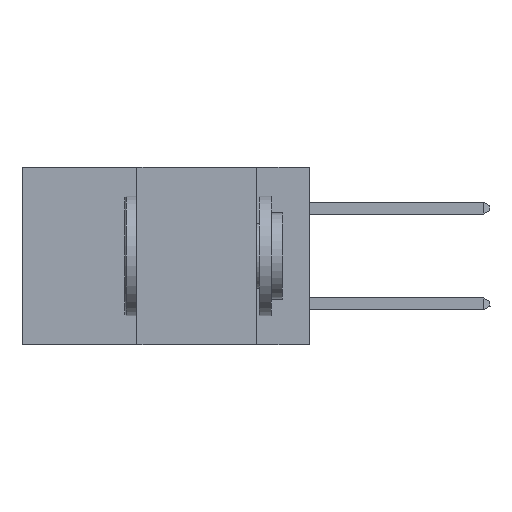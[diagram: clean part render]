
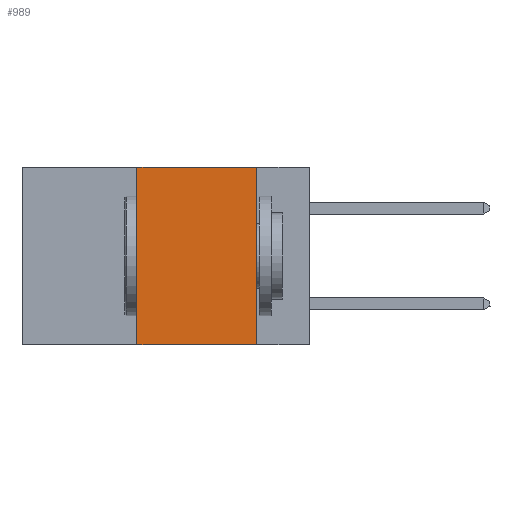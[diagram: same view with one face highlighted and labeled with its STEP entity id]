
A CAD part, left-side view. The second image highlights one B-rep face of the part: STEP entity #989.
In plain terms, the highlighted planar face has unit normal (-1, 0, 0).
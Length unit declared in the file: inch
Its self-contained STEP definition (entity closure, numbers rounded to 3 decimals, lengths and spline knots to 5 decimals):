
#76 = CARTESIAN_POINT ( 'NONE',  ( 0., 0.6, -0.37 ) ) ;
#334 = CARTESIAN_POINT ( 'NONE',  ( 0., 0.6, 0. ) ) ;
#580 = FACE_OUTER_BOUND ( 'NONE', #6560, .T. ) ;
#989 = ADVANCED_FACE ( 'NONE', ( #580 ), #5306, .F. ) ;
#1881 = DIRECTION ( 'NONE',  ( 0., -1., 0. ) ) ;
#2029 = CARTESIAN_POINT ( 'NONE',  ( 0., 0.11, -0.37 ) ) ;
#2171 = LINE ( 'NONE', #334, #7548 ) ;
#2260 = CARTESIAN_POINT ( 'NONE',  ( 0., 0.11, 0. ) ) ;
#2348 = DIRECTION ( 'NONE',  ( 0., 0., -1. ) ) ;
#2390 = CARTESIAN_POINT ( 'NONE',  ( 0., 0.6, 0. ) ) ;
#2432 = VERTEX_POINT ( 'NONE', #2260 ) ;
#2575 = AXIS2_PLACEMENT_3D ( 'NONE', #2390, #3129, #2348 ) ;
#2622 = ORIENTED_EDGE ( 'NONE', *, *, #2880, .F. ) ;
#2880 = EDGE_CURVE ( 'NONE', #8589, #2432, #2171, .T. ) ;
#3129 = DIRECTION ( 'NONE',  ( 1., 0., 0. ) ) ;
#3228 = VERTEX_POINT ( 'NONE', #2029 ) ;
#3977 = LINE ( 'NONE', #4073, #7385 ) ;
#4073 = CARTESIAN_POINT ( 'NONE',  ( 0., 0.36, 0. ) ) ;
#4931 = VECTOR ( 'NONE', #7813, 39.37008 ) ;
#5161 = EDGE_CURVE ( 'NONE', #2432, #3228, #7021, .T. ) ;
#5306 = PLANE ( 'NONE',  #2575 ) ;
#5912 = EDGE_CURVE ( 'NONE', #8092, #3228, #7150, .T. ) ;
#6020 = DIRECTION ( 'NONE',  ( 0., -1., 0. ) ) ;
#6100 = EDGE_CURVE ( 'NONE', #8092, #8589, #3977, .T. ) ;
#6308 = VECTOR ( 'NONE', #6020, 39.37008 ) ;
#6342 = ORIENTED_EDGE ( 'NONE', *, *, #5161, .F. ) ;
#6560 = EDGE_LOOP ( 'NONE', ( #6342, #2622, #9528, #8647 ) ) ;
#6980 = CARTESIAN_POINT ( 'NONE',  ( 0., 0.11, 0. ) ) ;
#7021 = LINE ( 'NONE', #6980, #4931 ) ;
#7150 = LINE ( 'NONE', #76, #6308 ) ;
#7385 = VECTOR ( 'NONE', #8739, 39.37008 ) ;
#7548 = VECTOR ( 'NONE', #1881, 39.37008 ) ;
#7813 = DIRECTION ( 'NONE',  ( 0., 0., -1. ) ) ;
#8092 = VERTEX_POINT ( 'NONE', #9526 ) ;
#8589 = VERTEX_POINT ( 'NONE', #9087 ) ;
#8647 = ORIENTED_EDGE ( 'NONE', *, *, #5912, .T. ) ;
#8739 = DIRECTION ( 'NONE',  ( 0., 0., 1. ) ) ;
#9087 = CARTESIAN_POINT ( 'NONE',  ( 0., 0.36, 0. ) ) ;
#9526 = CARTESIAN_POINT ( 'NONE',  ( 0., 0.36, -0.37 ) ) ;
#9528 = ORIENTED_EDGE ( 'NONE', *, *, #6100, .F. ) ;
